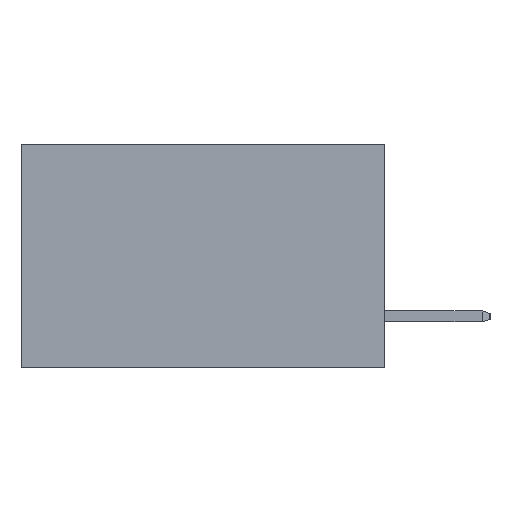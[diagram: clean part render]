
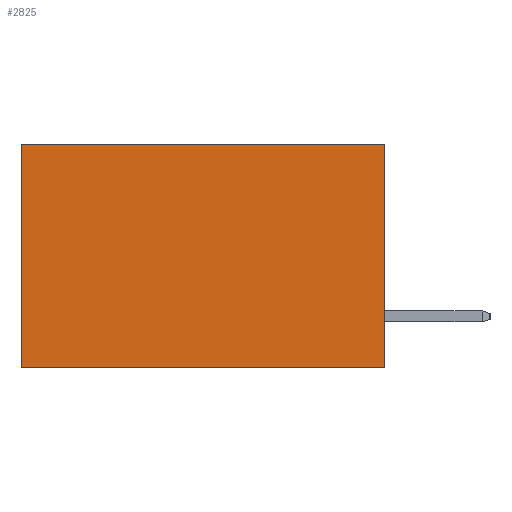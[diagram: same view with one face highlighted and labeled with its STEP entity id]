
A CAD part, left-side view. The second image highlights one B-rep face of the part: STEP entity #2825.
In plain terms, the highlighted planar face has unit normal (-1, 0, 0).
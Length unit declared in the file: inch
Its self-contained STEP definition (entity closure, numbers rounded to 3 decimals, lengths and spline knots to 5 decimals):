
#628 = EDGE_CURVE ( 'NONE', #4818, #10046, #5690, .T. ) ;
#800 = ORIENTED_EDGE ( 'NONE', *, *, #11455, .F. ) ;
#1098 = DIRECTION ( 'NONE',  ( 0., 1., 0. ) ) ;
#1158 = CARTESIAN_POINT ( 'NONE',  ( 0.2615, 0., 0. ) ) ;
#1939 = EDGE_CURVE ( 'NONE', #5746, #14002, #4791, .T. ) ;
#2432 = VECTOR ( 'NONE', #17729, 39.37008 ) ;
#2825 = ADVANCED_FACE ( 'NONE', ( #3094 ), #16504, .F. ) ;
#2900 = ORIENTED_EDGE ( 'NONE', *, *, #12649, .T. ) ;
#3094 = FACE_OUTER_BOUND ( 'NONE', #7767, .T. ) ;
#4285 = CARTESIAN_POINT ( 'NONE',  ( 0.2615, 0., -0.37 ) ) ;
#4791 = LINE ( 'NONE', #15233, #11186 ) ;
#4818 = VERTEX_POINT ( 'NONE', #10084 ) ;
#5690 = LINE ( 'NONE', #9325, #2432 ) ;
#5746 = VERTEX_POINT ( 'NONE', #15079 ) ;
#7067 = DIRECTION ( 'NONE',  ( 0., 0., -1. ) ) ;
#7418 = VECTOR ( 'NONE', #1098, 39.37008 ) ;
#7767 = EDGE_LOOP ( 'NONE', ( #14377, #800, #14933, #2900 ) ) ;
#8988 = VECTOR ( 'NONE', #16344, 39.37008 ) ;
#9291 = CARTESIAN_POINT ( 'NONE',  ( 0.2615, 0., -0.37 ) ) ;
#9325 = CARTESIAN_POINT ( 'NONE',  ( 0.2615, 0.6, -0.37 ) ) ;
#10046 = VERTEX_POINT ( 'NONE', #12259 ) ;
#10084 = CARTESIAN_POINT ( 'NONE',  ( 0.2615, 0.6, 0. ) ) ;
#11186 = VECTOR ( 'NONE', #15269, 39.37008 ) ;
#11455 = EDGE_CURVE ( 'NONE', #14002, #10046, #12634, .T. ) ;
#12259 = CARTESIAN_POINT ( 'NONE',  ( 0.2615, 0.6, -0.37 ) ) ;
#12634 = LINE ( 'NONE', #16591, #8988 ) ;
#12649 = EDGE_CURVE ( 'NONE', #5746, #4818, #17438, .T. ) ;
#14002 = VERTEX_POINT ( 'NONE', #4285 ) ;
#14377 = ORIENTED_EDGE ( 'NONE', *, *, #628, .T. ) ;
#14933 = ORIENTED_EDGE ( 'NONE', *, *, #1939, .F. ) ;
#15079 = CARTESIAN_POINT ( 'NONE',  ( 0.2615, 0., 0. ) ) ;
#15233 = CARTESIAN_POINT ( 'NONE',  ( 0.2615, 0., -0.37 ) ) ;
#15269 = DIRECTION ( 'NONE',  ( 0., 0., -1. ) ) ;
#16344 = DIRECTION ( 'NONE',  ( 0., 1., 0. ) ) ;
#16504 = PLANE ( 'NONE',  #17309 ) ;
#16591 = CARTESIAN_POINT ( 'NONE',  ( 0.2615, 0., -0.37 ) ) ;
#17240 = DIRECTION ( 'NONE',  ( 1., 0., 0. ) ) ;
#17309 = AXIS2_PLACEMENT_3D ( 'NONE', #9291, #17240, #7067 ) ;
#17438 = LINE ( 'NONE', #1158, #7418 ) ;
#17729 = DIRECTION ( 'NONE',  ( 0., 0., -1. ) ) ;
